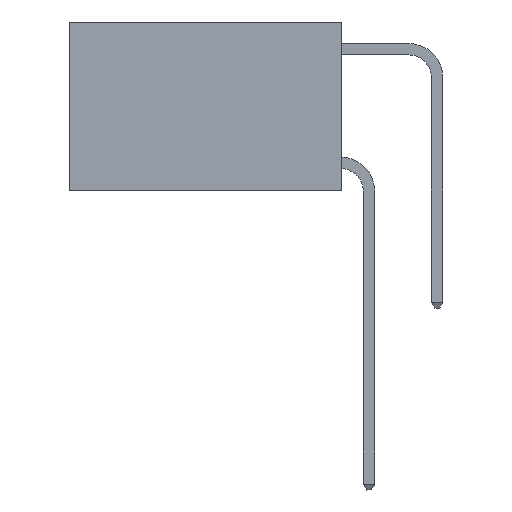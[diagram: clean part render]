
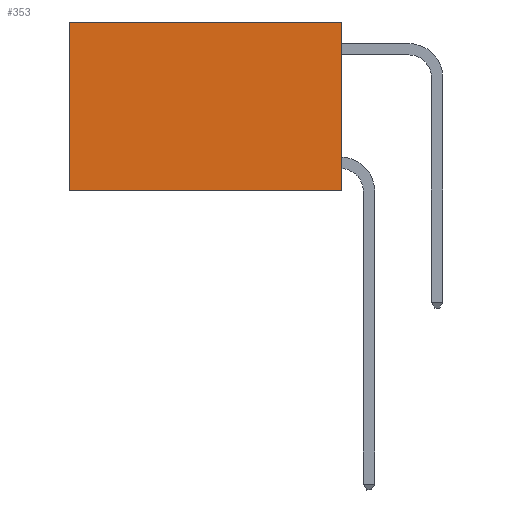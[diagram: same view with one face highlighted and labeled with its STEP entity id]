
A CAD part, left-side view. The second image highlights one B-rep face of the part: STEP entity #353.
In plain terms, the highlighted planar face has unit normal (-1, 0, 0).
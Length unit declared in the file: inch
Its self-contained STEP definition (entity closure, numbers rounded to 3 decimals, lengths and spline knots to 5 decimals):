
#263 = CARTESIAN_POINT ( 'NONE',  ( 0.2625, 0.6, 0. ) ) ;
#275 = VECTOR ( 'NONE', #1577, 39.37008 ) ;
#281 = ORIENTED_EDGE ( 'NONE', *, *, #3806, .F. ) ;
#353 = ADVANCED_FACE ( 'NONE', ( #2954 ), #5994, .F. ) ;
#540 = CARTESIAN_POINT ( 'NONE',  ( 0.2625, 0., 0. ) ) ;
#590 = CARTESIAN_POINT ( 'NONE',  ( 0.2625, 0., 0. ) ) ;
#737 = LINE ( 'NONE', #540, #8961 ) ;
#739 = VECTOR ( 'NONE', #5336, 39.37008 ) ;
#1202 = DIRECTION ( 'NONE',  ( 0., 1., 0. ) ) ;
#1577 = DIRECTION ( 'NONE',  ( 0., 0., -1. ) ) ;
#1775 = VECTOR ( 'NONE', #1202, 39.37008 ) ;
#2042 = VERTEX_POINT ( 'NONE', #8985 ) ;
#2056 = AXIS2_PLACEMENT_3D ( 'NONE', #9237, #3200, #8385 ) ;
#2131 = CARTESIAN_POINT ( 'NONE',  ( 0.2625, 0., -0.37 ) ) ;
#2954 = FACE_OUTER_BOUND ( 'NONE', #4571, .T. ) ;
#3200 = DIRECTION ( 'NONE',  ( 1., 0., 0. ) ) ;
#3290 = CARTESIAN_POINT ( 'NONE',  ( 0.2625, 0., 0. ) ) ;
#3806 = EDGE_CURVE ( 'NONE', #8062, #2042, #4469, .T. ) ;
#4024 = EDGE_CURVE ( 'NONE', #5310, #2042, #9171, .T. ) ;
#4469 = LINE ( 'NONE', #2131, #739 ) ;
#4571 = EDGE_LOOP ( 'NONE', ( #6976, #281, #5693, #9541 ) ) ;
#5260 = DIRECTION ( 'NONE',  ( 0., 0., -1. ) ) ;
#5310 = VERTEX_POINT ( 'NONE', #7672 ) ;
#5336 = DIRECTION ( 'NONE',  ( 0., 1., 0. ) ) ;
#5693 = ORIENTED_EDGE ( 'NONE', *, *, #9247, .F. ) ;
#5994 = PLANE ( 'NONE',  #2056 ) ;
#6976 = ORIENTED_EDGE ( 'NONE', *, *, #4024, .T. ) ;
#7202 = LINE ( 'NONE', #3290, #1775 ) ;
#7672 = CARTESIAN_POINT ( 'NONE',  ( 0.2625, 0.6, 0. ) ) ;
#8018 = EDGE_CURVE ( 'NONE', #9239, #5310, #7202, .T. ) ;
#8062 = VERTEX_POINT ( 'NONE', #9028 ) ;
#8385 = DIRECTION ( 'NONE',  ( 0., 0., -1. ) ) ;
#8961 = VECTOR ( 'NONE', #5260, 39.37008 ) ;
#8985 = CARTESIAN_POINT ( 'NONE',  ( 0.2625, 0.6, -0.37 ) ) ;
#9028 = CARTESIAN_POINT ( 'NONE',  ( 0.2625, 0., -0.37 ) ) ;
#9171 = LINE ( 'NONE', #263, #275 ) ;
#9237 = CARTESIAN_POINT ( 'NONE',  ( 0.2625, 0., 0. ) ) ;
#9239 = VERTEX_POINT ( 'NONE', #590 ) ;
#9247 = EDGE_CURVE ( 'NONE', #9239, #8062, #737, .T. ) ;
#9541 = ORIENTED_EDGE ( 'NONE', *, *, #8018, .T. ) ;
